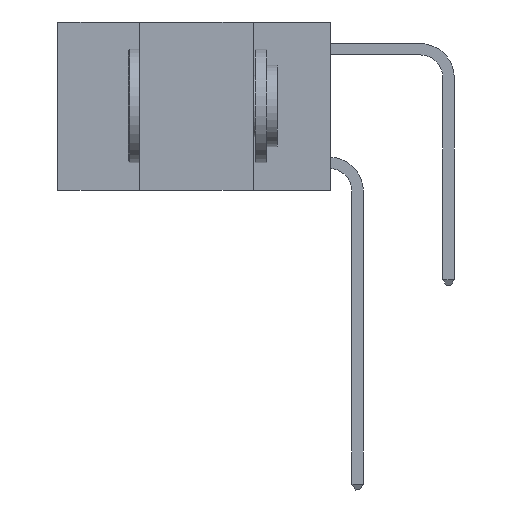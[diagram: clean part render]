
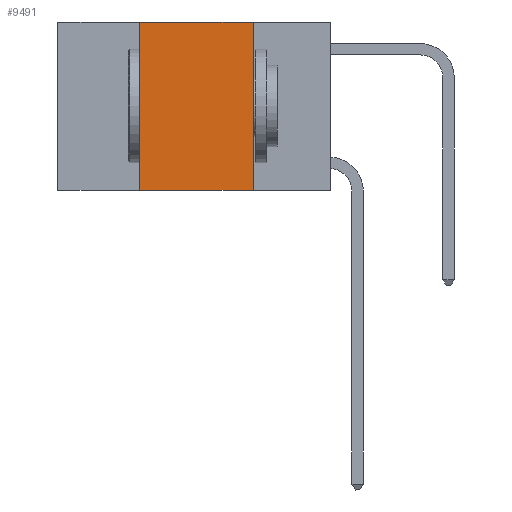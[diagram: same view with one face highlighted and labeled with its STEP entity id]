
A CAD part, left-side view. The second image highlights one B-rep face of the part: STEP entity #9491.
In plain terms, the highlighted planar face has unit normal (-1, 0, 0).
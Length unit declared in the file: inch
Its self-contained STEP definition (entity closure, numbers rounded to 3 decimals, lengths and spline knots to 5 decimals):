
#33 = LINE ( 'NONE', #5173, #88 ) ;
#88 = VECTOR ( 'NONE', #896, 39.37008 ) ;
#310 = DIRECTION ( 'NONE',  ( 1., 0., 0. ) ) ;
#392 = VECTOR ( 'NONE', #5296, 39.37008 ) ;
#417 = CARTESIAN_POINT ( 'NONE',  ( 0., 0.42, -0.37 ) ) ;
#896 = DIRECTION ( 'NONE',  ( 0., -1., 0. ) ) ;
#1321 = ORIENTED_EDGE ( 'NONE', *, *, #9291, .F. ) ;
#1474 = VECTOR ( 'NONE', #7504, 39.37008 ) ;
#1763 = DIRECTION ( 'NONE',  ( 0., -1., 0. ) ) ;
#2675 = CARTESIAN_POINT ( 'NONE',  ( 0., 0.17, 0. ) ) ;
#2976 = CARTESIAN_POINT ( 'NONE',  ( 0., 0.42, 0. ) ) ;
#3366 = VERTEX_POINT ( 'NONE', #8478 ) ;
#3780 = EDGE_CURVE ( 'NONE', #5996, #3366, #7698, .T. ) ;
#3938 = EDGE_CURVE ( 'NONE', #4517, #9670, #5407, .T. ) ;
#4417 = CARTESIAN_POINT ( 'NONE',  ( 0., 0.42, 0. ) ) ;
#4517 = VERTEX_POINT ( 'NONE', #417 ) ;
#4645 = FACE_OUTER_BOUND ( 'NONE', #11122, .T. ) ;
#5173 = CARTESIAN_POINT ( 'NONE',  ( 0., 0.6, 0. ) ) ;
#5296 = DIRECTION ( 'NONE',  ( 0., 0., -1. ) ) ;
#5407 = LINE ( 'NONE', #2976, #1474 ) ;
#5996 = VERTEX_POINT ( 'NONE', #2675 ) ;
#7437 = EDGE_CURVE ( 'NONE', #4517, #3366, #9667, .T. ) ;
#7504 = DIRECTION ( 'NONE',  ( 0., 0., 1. ) ) ;
#7698 = LINE ( 'NONE', #11276, #392 ) ;
#8149 = PLANE ( 'NONE',  #8447 ) ;
#8447 = AXIS2_PLACEMENT_3D ( 'NONE', #9685, #310, #9917 ) ;
#8478 = CARTESIAN_POINT ( 'NONE',  ( 0., 0.17, -0.37 ) ) ;
#8678 = ORIENTED_EDGE ( 'NONE', *, *, #7437, .T. ) ;
#8810 = CARTESIAN_POINT ( 'NONE',  ( 0., 0.6, -0.37 ) ) ;
#9291 = EDGE_CURVE ( 'NONE', #9670, #5996, #33, .T. ) ;
#9457 = ORIENTED_EDGE ( 'NONE', *, *, #3780, .F. ) ;
#9491 = ADVANCED_FACE ( 'NONE', ( #4645 ), #8149, .F. ) ;
#9667 = LINE ( 'NONE', #8810, #10904 ) ;
#9670 = VERTEX_POINT ( 'NONE', #4417 ) ;
#9685 = CARTESIAN_POINT ( 'NONE',  ( 0., 0.6, 0. ) ) ;
#9917 = DIRECTION ( 'NONE',  ( 0., 0., -1. ) ) ;
#10806 = ORIENTED_EDGE ( 'NONE', *, *, #3938, .F. ) ;
#10904 = VECTOR ( 'NONE', #1763, 39.37008 ) ;
#11122 = EDGE_LOOP ( 'NONE', ( #9457, #1321, #10806, #8678 ) ) ;
#11276 = CARTESIAN_POINT ( 'NONE',  ( 0., 0.17, 0. ) ) ;
